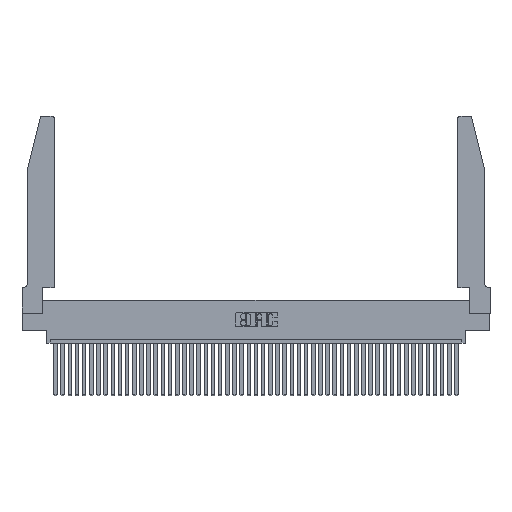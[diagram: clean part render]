
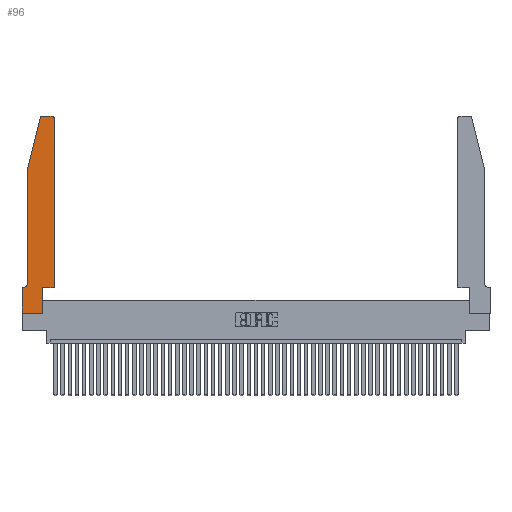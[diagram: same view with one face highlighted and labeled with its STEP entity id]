
A CAD part, top view. The second image highlights one B-rep face of the part: STEP entity #96.
In plain terms, the highlighted planar face has unit normal (0, 0, 1).
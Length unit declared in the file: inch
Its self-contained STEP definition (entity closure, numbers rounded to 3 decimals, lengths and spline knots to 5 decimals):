
#96 = ADVANCED_FACE ( 'NONE', ( #35886 ), #30223, .T. ) ;
#181 = ORIENTED_EDGE ( 'NONE', *, *, #10885, .T. ) ;
#383 = VECTOR ( 'NONE', #45068, 39.37008 ) ;
#1687 = VERTEX_POINT ( 'NONE', #6821 ) ;
#1835 = EDGE_LOOP ( 'NONE', ( #17184, #22139, #5407, #18608, #8058, #181, #28815, #42901, #19188, #30062, #6322, #32927 ) ) ;
#2030 = CARTESIAN_POINT ( 'NONE',  ( 0.0755, 2., 0.37 ) ) ;
#2234 = VECTOR ( 'NONE', #20656, 39.37008 ) ;
#2720 = CARTESIAN_POINT ( 'NONE',  ( 0., 0.35, 0.37 ) ) ;
#4506 = CARTESIAN_POINT ( 'NONE',  ( 0.284, 2.72, 0.37 ) ) ;
#4777 = LINE ( 'NONE', #42443, #41154 ) ;
#4844 = EDGE_CURVE ( 'NONE', #1687, #37281, #4777, .T. ) ;
#5137 = VERTEX_POINT ( 'NONE', #37798 ) ;
#5407 = ORIENTED_EDGE ( 'NONE', *, *, #36029, .T. ) ;
#6322 = ORIENTED_EDGE ( 'NONE', *, *, #32164, .T. ) ;
#6708 = LINE ( 'NONE', #41776, #2234 ) ;
#6821 = CARTESIAN_POINT ( 'NONE',  ( 0.2865, 0.35, 0.37 ) ) ;
#7154 = CIRCLE ( 'NONE', #25598, 0.03 ) ;
#7512 = CARTESIAN_POINT ( 'NONE',  ( 0.4505, 0.35, 0.37 ) ) ;
#7651 = LINE ( 'NONE', #43306, #34704 ) ;
#8058 = ORIENTED_EDGE ( 'NONE', *, *, #32053, .T. ) ;
#8140 = DIRECTION ( 'NONE',  ( 0., 0., -1. ) ) ;
#8433 = VERTEX_POINT ( 'NONE', #41254 ) ;
#9409 = DIRECTION ( 'NONE',  ( -1., 0., 0. ) ) ;
#9641 = CIRCLE ( 'NONE', #23164, 0.07 ) ;
#10034 = CARTESIAN_POINT ( 'NONE',  ( 0.0755, 0.35, 0.37 ) ) ;
#10323 = CARTESIAN_POINT ( 'NONE',  ( 0.0755, 2., 0.37 ) ) ;
#10338 = CARTESIAN_POINT ( 'NONE',  ( 0., 0., 0.37 ) ) ;
#10878 = VERTEX_POINT ( 'NONE', #10338 ) ;
#10885 = EDGE_CURVE ( 'NONE', #23651, #24368, #41313, .T. ) ;
#11140 = EDGE_CURVE ( 'NONE', #35612, #45030, #31404, .T. ) ;
#11465 = DIRECTION ( 'NONE',  ( 1., 0., 0. ) ) ;
#11982 = EDGE_CURVE ( 'NONE', #10878, #27450, #38438, .T. ) ;
#12910 = VECTOR ( 'NONE', #37485, 39.37008 ) ;
#13386 = LINE ( 'NONE', #10323, #34874 ) ;
#13639 = CIRCLE ( 'NONE', #24470, 0.03 ) ;
#14782 = VERTEX_POINT ( 'NONE', #31393 ) ;
#15821 = VECTOR ( 'NONE', #43326, 39.37008 ) ;
#17184 = ORIENTED_EDGE ( 'NONE', *, *, #21599, .T. ) ;
#17650 = VERTEX_POINT ( 'NONE', #27445 ) ;
#18608 = ORIENTED_EDGE ( 'NONE', *, *, #11140, .T. ) ;
#18871 = CARTESIAN_POINT ( 'NONE',  ( 0.0755, 0.42, 0.37 ) ) ;
#19188 = ORIENTED_EDGE ( 'NONE', *, *, #37041, .T. ) ;
#20126 = CARTESIAN_POINT ( 'NONE',  ( 0.2865, 0., 0.37 ) ) ;
#20656 = DIRECTION ( 'NONE',  ( 0., 1., 0. ) ) ;
#21599 = EDGE_CURVE ( 'NONE', #8433, #14782, #35199, .T. ) ;
#22139 = ORIENTED_EDGE ( 'NONE', *, *, #37741, .T. ) ;
#23164 = AXIS2_PLACEMENT_3D ( 'NONE', #39632, #8140, #9409 ) ;
#23651 = VERTEX_POINT ( 'NONE', #26542 ) ;
#24090 = DIRECTION ( 'NONE',  ( -1., 0., 0. ) ) ;
#24108 = AXIS2_PLACEMENT_3D ( 'NONE', #34407, #43160, #29173 ) ;
#24368 = VERTEX_POINT ( 'NONE', #2720 ) ;
#24470 = AXIS2_PLACEMENT_3D ( 'NONE', #40670, #26674, #44224 ) ;
#25598 = AXIS2_PLACEMENT_3D ( 'NONE', #4506, #29296, #11465 ) ;
#26363 = VECTOR ( 'NONE', #24090, 39.37008 ) ;
#26542 = CARTESIAN_POINT ( 'NONE',  ( 0.0055, 0.35, 0.37 ) ) ;
#26674 = DIRECTION ( 'NONE',  ( 0., 0., 1. ) ) ;
#27445 = CARTESIAN_POINT ( 'NONE',  ( 0.4505, 2.72, 0.37 ) ) ;
#27450 = VERTEX_POINT ( 'NONE', #20126 ) ;
#28021 = CARTESIAN_POINT ( 'NONE',  ( 0.0755, 2., 0.37 ) ) ;
#28775 = CARTESIAN_POINT ( 'NONE',  ( 0., 0., 0.37 ) ) ;
#28815 = ORIENTED_EDGE ( 'NONE', *, *, #40084, .T. ) ;
#29173 = DIRECTION ( 'NONE',  ( 1., 0., 0. ) ) ;
#29296 = DIRECTION ( 'NONE',  ( 0., 0., 1. ) ) ;
#30062 = ORIENTED_EDGE ( 'NONE', *, *, #4844, .T. ) ;
#30223 = PLANE ( 'NONE',  #24108 ) ;
#30818 = VECTOR ( 'NONE', #34118, 39.37008 ) ;
#31059 = DIRECTION ( 'NONE',  ( -0.239, -0.971, 0. ) ) ;
#31259 = CARTESIAN_POINT ( 'NONE',  ( 0.2605, 2.75, 0.37 ) ) ;
#31303 = DIRECTION ( 'NONE',  ( 1., 0., 0. ) ) ;
#31393 = CARTESIAN_POINT ( 'NONE',  ( 0.284, 2.75, 0.37 ) ) ;
#31404 = LINE ( 'NONE', #2030, #30818 ) ;
#32053 = EDGE_CURVE ( 'NONE', #45030, #23651, #9641, .T. ) ;
#32164 = EDGE_CURVE ( 'NONE', #37281, #17650, #33231, .T. ) ;
#32927 = ORIENTED_EDGE ( 'NONE', *, *, #38722, .T. ) ;
#33231 = LINE ( 'NONE', #41164, #12910 ) ;
#34118 = DIRECTION ( 'NONE',  ( 0., -1., 0. ) ) ;
#34407 = CARTESIAN_POINT ( 'NONE',  ( 0., 0.35, 0.37 ) ) ;
#34704 = VECTOR ( 'NONE', #36567, 39.37008 ) ;
#34874 = VECTOR ( 'NONE', #31059, 39.37008 ) ;
#35199 = LINE ( 'NONE', #31259, #383 ) ;
#35612 = VERTEX_POINT ( 'NONE', #28021 ) ;
#35886 = FACE_OUTER_BOUND ( 'NONE', #1835, .T. ) ;
#36029 = EDGE_CURVE ( 'NONE', #5137, #35612, #13386, .T. ) ;
#36567 = DIRECTION ( 'NONE',  ( 0., -1., 0. ) ) ;
#37041 = EDGE_CURVE ( 'NONE', #27450, #1687, #6708, .T. ) ;
#37281 = VERTEX_POINT ( 'NONE', #7512 ) ;
#37485 = DIRECTION ( 'NONE',  ( 0., 1., 0. ) ) ;
#37741 = EDGE_CURVE ( 'NONE', #14782, #5137, #7154, .T. ) ;
#37798 = CARTESIAN_POINT ( 'NONE',  ( 0.25487, 2.72718, 0.37 ) ) ;
#38438 = LINE ( 'NONE', #28775, #15821 ) ;
#38722 = EDGE_CURVE ( 'NONE', #17650, #8433, #13639, .T. ) ;
#39632 = CARTESIAN_POINT ( 'NONE',  ( 0.0055, 0.42, 0.37 ) ) ;
#40084 = EDGE_CURVE ( 'NONE', #24368, #10878, #7651, .T. ) ;
#40670 = CARTESIAN_POINT ( 'NONE',  ( 0.4205, 2.72, 0.37 ) ) ;
#41154 = VECTOR ( 'NONE', #31303, 39.37008 ) ;
#41164 = CARTESIAN_POINT ( 'NONE',  ( 0.4505, 0.35, 0.37 ) ) ;
#41254 = CARTESIAN_POINT ( 'NONE',  ( 0.4205, 2.75, 0.37 ) ) ;
#41313 = LINE ( 'NONE', #10034, #26363 ) ;
#41776 = CARTESIAN_POINT ( 'NONE',  ( 0.2865, 0.35, 0.37 ) ) ;
#42443 = CARTESIAN_POINT ( 'NONE',  ( 0.4505, 0.35, 0.37 ) ) ;
#42901 = ORIENTED_EDGE ( 'NONE', *, *, #11982, .T. ) ;
#43160 = DIRECTION ( 'NONE',  ( 0., 0., 1. ) ) ;
#43306 = CARTESIAN_POINT ( 'NONE',  ( 0., 0., 0.37 ) ) ;
#43326 = DIRECTION ( 'NONE',  ( 1., 0., 0. ) ) ;
#44224 = DIRECTION ( 'NONE',  ( 1., 0., 0. ) ) ;
#45030 = VERTEX_POINT ( 'NONE', #18871 ) ;
#45068 = DIRECTION ( 'NONE',  ( -1., 0., 0. ) ) ;
